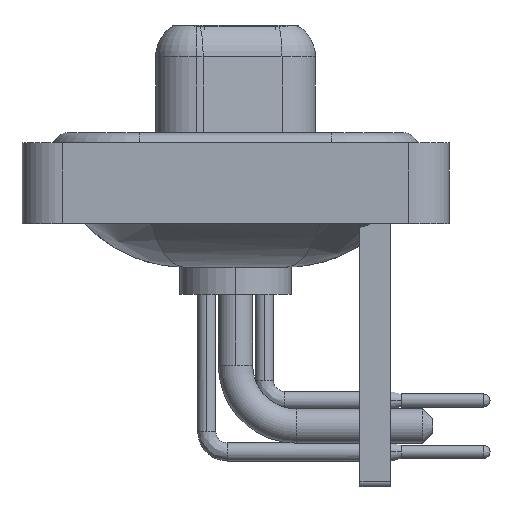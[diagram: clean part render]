
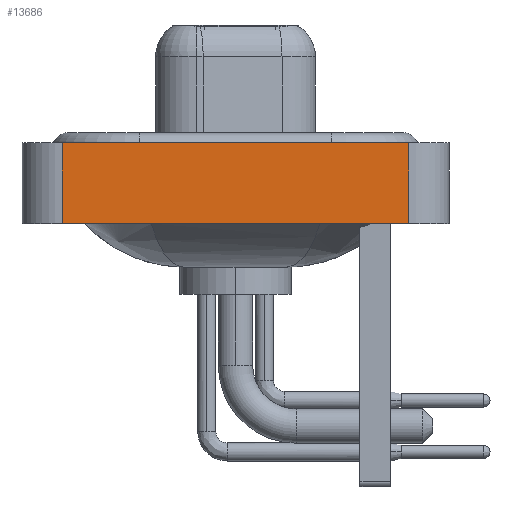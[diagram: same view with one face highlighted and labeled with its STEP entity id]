
A CAD part, left-side view. The second image highlights one B-rep face of the part: STEP entity #13686.
In plain terms, the highlighted planar face has unit normal (-1, 0, 0).
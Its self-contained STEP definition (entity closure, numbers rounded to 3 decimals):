
#81 = LINE ( 'NONE', #19984, #18977 ) ;
#90 = CARTESIAN_POINT ( 'NONE',  ( -7.3, -8.55, 0.4 ) ) ;
#909 = LINE ( 'NONE', #5658, #19810 ) ;
#1222 = EDGE_CURVE ( 'NONE', #12358, #13300, #9997, .T. ) ;
#1591 = VERTEX_POINT ( 'NONE', #6989 ) ;
#1670 = CARTESIAN_POINT ( 'NONE',  ( -7.3, 8.55, 0.4 ) ) ;
#1671 = EDGE_CURVE ( 'NONE', #1591, #9138, #18795, .T. ) ;
#1913 = DIRECTION ( 'NONE',  ( 0., 0., 1. ) ) ;
#2083 = ORIENTED_EDGE ( 'NONE', *, *, #1222, .F. ) ;
#2298 = EDGE_CURVE ( 'NONE', #13300, #9138, #909, .T. ) ;
#5164 = DIRECTION ( 'NONE',  ( 0., -1., 0. ) ) ;
#5658 = CARTESIAN_POINT ( 'NONE',  ( -7.3, -8.55, 0.4 ) ) ;
#5955 = VECTOR ( 'NONE', #1913, 1000. ) ;
#6989 = CARTESIAN_POINT ( 'NONE',  ( -7.3, -8.55, -3.6 ) ) ;
#7499 = CARTESIAN_POINT ( 'NONE',  ( -7.3, 8.55, -3.6 ) ) ;
#7503 = ORIENTED_EDGE ( 'NONE', *, *, #1671, .T. ) ;
#8106 = DIRECTION ( 'NONE',  ( -1., 0., 0. ) ) ;
#8320 = FACE_OUTER_BOUND ( 'NONE', #8820, .T. ) ;
#8820 = EDGE_LOOP ( 'NONE', ( #7503, #9024, #2083, #18194 ) ) ;
#9024 = ORIENTED_EDGE ( 'NONE', *, *, #2298, .F. ) ;
#9138 = VERTEX_POINT ( 'NONE', #90 ) ;
#9353 = DIRECTION ( 'NONE',  ( 0., -1., 0. ) ) ;
#9997 = LINE ( 'NONE', #14961, #14942 ) ;
#10588 = AXIS2_PLACEMENT_3D ( 'NONE', #13403, #8106, #13087 ) ;
#12358 = VERTEX_POINT ( 'NONE', #7499 ) ;
#13087 = DIRECTION ( 'NONE',  ( 0., 0., 1. ) ) ;
#13189 = PLANE ( 'NONE',  #10588 ) ;
#13300 = VERTEX_POINT ( 'NONE', #1670 ) ;
#13403 = CARTESIAN_POINT ( 'NONE',  ( -7.3, -8.55, -3.6 ) ) ;
#13686 = ADVANCED_FACE ( 'NONE', ( #8320 ), #13189, .T. ) ;
#14942 = VECTOR ( 'NONE', #19941, 1000. ) ;
#14961 = CARTESIAN_POINT ( 'NONE',  ( -7.3, 8.55, -3.6 ) ) ;
#15399 = EDGE_CURVE ( 'NONE', #12358, #1591, #81, .T. ) ;
#15554 = CARTESIAN_POINT ( 'NONE',  ( -7.3, -8.55, -3.6 ) ) ;
#18194 = ORIENTED_EDGE ( 'NONE', *, *, #15399, .T. ) ;
#18795 = LINE ( 'NONE', #15554, #5955 ) ;
#18977 = VECTOR ( 'NONE', #5164, 1000. ) ;
#19810 = VECTOR ( 'NONE', #9353, 1000. ) ;
#19941 = DIRECTION ( 'NONE',  ( 0., 0., 1. ) ) ;
#19984 = CARTESIAN_POINT ( 'NONE',  ( -7.3, -8.55, -3.6 ) ) ;
